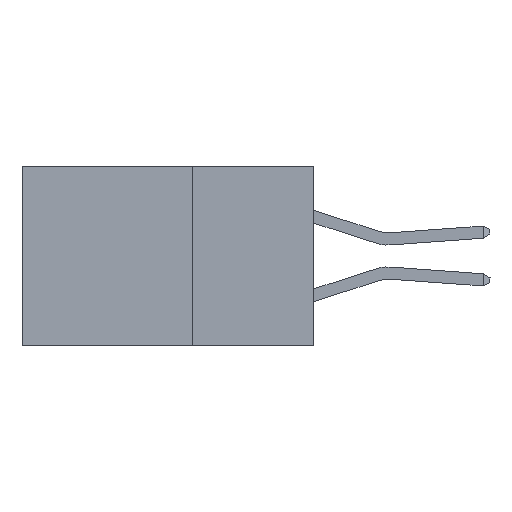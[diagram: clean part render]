
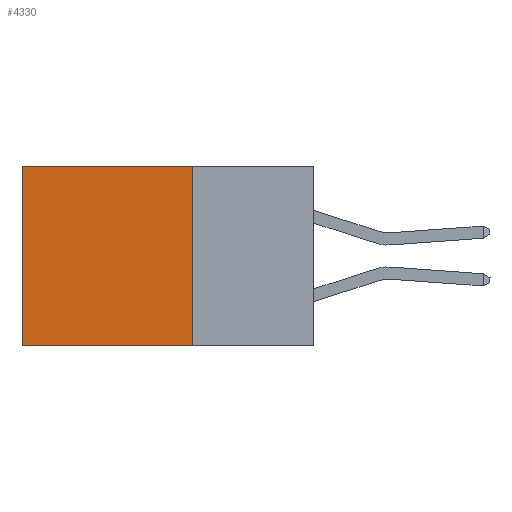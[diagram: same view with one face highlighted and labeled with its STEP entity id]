
A CAD part, left-side view. The second image highlights one B-rep face of the part: STEP entity #4330.
In plain terms, the highlighted planar face has unit normal (-1, 0, 0).
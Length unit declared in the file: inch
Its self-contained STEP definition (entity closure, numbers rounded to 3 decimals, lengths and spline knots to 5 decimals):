
#652 = VECTOR ( 'NONE', #2895, 39.37008 ) ;
#1136 = DIRECTION ( 'NONE',  ( 0., 1., 0. ) ) ;
#1533 = ORIENTED_EDGE ( 'NONE', *, *, #22094, .T. ) ;
#2161 = VECTOR ( 'NONE', #1136, 39.37008 ) ;
#2895 = DIRECTION ( 'NONE',  ( 0., 1., 0. ) ) ;
#3151 = VECTOR ( 'NONE', #25626, 39.37008 ) ;
#4330 = ADVANCED_FACE ( 'NONE', ( #26765 ), #8315, .F. ) ;
#4956 = EDGE_CURVE ( 'NONE', #43977, #21656, #20310, .T. ) ;
#6748 = CARTESIAN_POINT ( 'NONE',  ( 0.2875, 0.25, 0. ) ) ;
#7997 = CARTESIAN_POINT ( 'NONE',  ( 0.2875, 0.25, -0.37 ) ) ;
#8315 = PLANE ( 'NONE',  #19674 ) ;
#18461 = VECTOR ( 'NONE', #20493, 39.37008 ) ;
#18618 = DIRECTION ( 'NONE',  ( 1., 0., 0. ) ) ;
#18633 = EDGE_CURVE ( 'NONE', #42814, #23063, #28948, .T. ) ;
#19674 = AXIS2_PLACEMENT_3D ( 'NONE', #39026, #18618, #42451 ) ;
#20310 = LINE ( 'NONE', #24989, #2161 ) ;
#20493 = DIRECTION ( 'NONE',  ( 0., 0., -1. ) ) ;
#20964 = ORIENTED_EDGE ( 'NONE', *, *, #38079, .F. ) ;
#21656 = VERTEX_POINT ( 'NONE', #40556 ) ;
#22094 = EDGE_CURVE ( 'NONE', #21656, #23063, #30382, .T. ) ;
#23063 = VERTEX_POINT ( 'NONE', #42326 ) ;
#24989 = CARTESIAN_POINT ( 'NONE',  ( 0.2875, 0.25, 0. ) ) ;
#25626 = DIRECTION ( 'NONE',  ( 0., 0., -1. ) ) ;
#26765 = FACE_OUTER_BOUND ( 'NONE', #31141, .T. ) ;
#28618 = LINE ( 'NONE', #6748, #18461 ) ;
#28948 = LINE ( 'NONE', #43723, #652 ) ;
#29699 = CARTESIAN_POINT ( 'NONE',  ( 0.2875, 0.25, 0. ) ) ;
#30382 = LINE ( 'NONE', #39172, #3151 ) ;
#30712 = ORIENTED_EDGE ( 'NONE', *, *, #4956, .T. ) ;
#31141 = EDGE_LOOP ( 'NONE', ( #1533, #32017, #20964, #30712 ) ) ;
#32017 = ORIENTED_EDGE ( 'NONE', *, *, #18633, .F. ) ;
#38079 = EDGE_CURVE ( 'NONE', #43977, #42814, #28618, .T. ) ;
#39026 = CARTESIAN_POINT ( 'NONE',  ( 0.2875, 0.25, 0. ) ) ;
#39172 = CARTESIAN_POINT ( 'NONE',  ( 0.2875, 0.6, 0. ) ) ;
#40556 = CARTESIAN_POINT ( 'NONE',  ( 0.2875, 0.6, 0. ) ) ;
#42326 = CARTESIAN_POINT ( 'NONE',  ( 0.2875, 0.6, -0.37 ) ) ;
#42451 = DIRECTION ( 'NONE',  ( 0., 0., -1. ) ) ;
#42814 = VERTEX_POINT ( 'NONE', #7997 ) ;
#43723 = CARTESIAN_POINT ( 'NONE',  ( 0.2875, 0.25, -0.37 ) ) ;
#43977 = VERTEX_POINT ( 'NONE', #29699 ) ;
